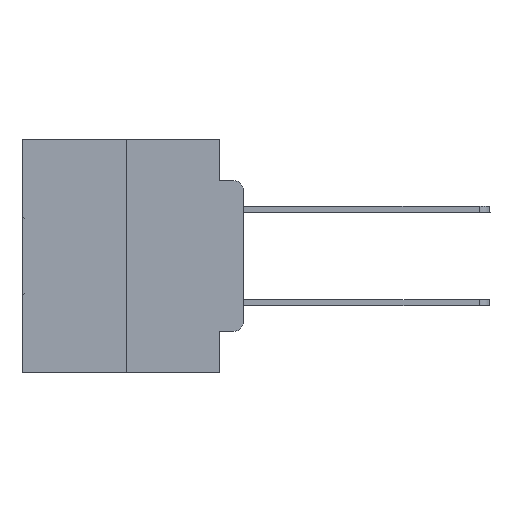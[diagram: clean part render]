
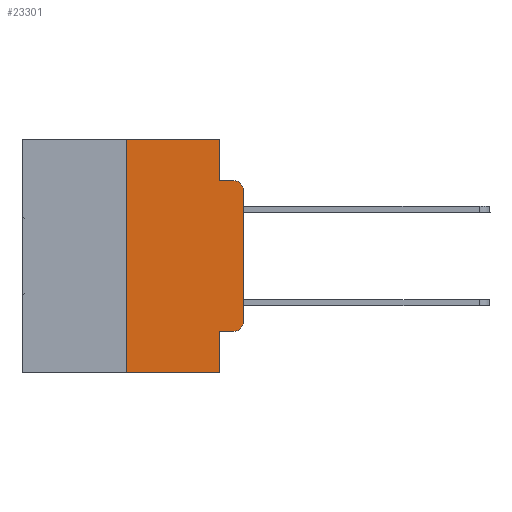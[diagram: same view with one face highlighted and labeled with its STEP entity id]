
A CAD part, left-side view. The second image highlights one B-rep face of the part: STEP entity #23301.
In plain terms, the highlighted planar face has unit normal (-1, 0, 0).
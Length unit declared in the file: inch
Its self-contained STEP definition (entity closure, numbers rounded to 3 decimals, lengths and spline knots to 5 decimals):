
#1292 = DIRECTION ( 'NONE',  ( 0., -1., 0. ) ) ;
#1364 = VECTOR ( 'NONE', #5255, 39.37008 ) ;
#1544 = AXIS2_PLACEMENT_3D ( 'NONE', #30973, #25988, #23099 ) ;
#1579 = VERTEX_POINT ( 'NONE', #13675 ) ;
#2563 = AXIS2_PLACEMENT_3D ( 'NONE', #10054, #17796, #10563 ) ;
#2618 = AXIS2_PLACEMENT_3D ( 'NONE', #30300, #25302, #14873 ) ;
#2721 = CARTESIAN_POINT ( 'NONE',  ( 0., 0.051, -0.4115 ) ) ;
#3250 = ORIENTED_EDGE ( 'NONE', *, *, #9442, .T. ) ;
#3460 = LINE ( 'NONE', #6198, #9876 ) ;
#3686 = VECTOR ( 'NONE', #20062, 39.37008 ) ;
#4103 = CARTESIAN_POINT ( 'NONE',  ( 0., 0.25, 0. ) ) ;
#4398 = LINE ( 'NONE', #9399, #3686 ) ;
#4515 = VERTEX_POINT ( 'NONE', #13543 ) ;
#4553 = CARTESIAN_POINT ( 'NONE',  ( 0., 0.473, 0. ) ) ;
#4576 = CARTESIAN_POINT ( 'NONE',  ( 0., 0.051, 0. ) ) ;
#4718 = EDGE_CURVE ( 'NONE', #13504, #28247, #10781, .T. ) ;
#4953 = CARTESIAN_POINT ( 'NONE',  ( 0., 0.051, -0.0885 ) ) ;
#5255 = DIRECTION ( 'NONE',  ( 0., 0., -1. ) ) ;
#5365 = CIRCLE ( 'NONE', #2618, 0.02 ) ;
#6198 = CARTESIAN_POINT ( 'NONE',  ( 0., 0.051, -0.0885 ) ) ;
#6205 = VECTOR ( 'NONE', #6881, 39.37008 ) ;
#6881 = DIRECTION ( 'NONE',  ( 0., 0., 1. ) ) ;
#7308 = DIRECTION ( 'NONE',  ( 0., -1., 0. ) ) ;
#7390 = EDGE_CURVE ( 'NONE', #4515, #11070, #23462, .T. ) ;
#7546 = EDGE_CURVE ( 'NONE', #19605, #24317, #3460, .T. ) ;
#8857 = LINE ( 'NONE', #2721, #30768 ) ;
#8997 = ORIENTED_EDGE ( 'NONE', *, *, #23970, .F. ) ;
#9291 = CARTESIAN_POINT ( 'NONE',  ( 0., 0.02, -0.4115 ) ) ;
#9399 = CARTESIAN_POINT ( 'NONE',  ( 0., 0.051, 0. ) ) ;
#9401 = ORIENTED_EDGE ( 'NONE', *, *, #23253, .T. ) ;
#9442 = EDGE_CURVE ( 'NONE', #4515, #11794, #11894, .T. ) ;
#9876 = VECTOR ( 'NONE', #13974, 39.37008 ) ;
#10054 = CARTESIAN_POINT ( 'NONE',  ( 0., 0.02, -0.3915 ) ) ;
#10563 = DIRECTION ( 'NONE',  ( 0., 0., -1. ) ) ;
#10646 = EDGE_CURVE ( 'NONE', #28247, #1579, #32330, .T. ) ;
#10781 = CIRCLE ( 'NONE', #2563, 0.02 ) ;
#11038 = DIRECTION ( 'NONE',  ( 0., 0., 1. ) ) ;
#11070 = VERTEX_POINT ( 'NONE', #4103 ) ;
#11562 = CARTESIAN_POINT ( 'NONE',  ( 0., 0., 0. ) ) ;
#11794 = VERTEX_POINT ( 'NONE', #12230 ) ;
#11894 = LINE ( 'NONE', #27161, #32446 ) ;
#12230 = CARTESIAN_POINT ( 'NONE',  ( 0., 0.051, -0.5 ) ) ;
#13504 = VERTEX_POINT ( 'NONE', #9291 ) ;
#13543 = CARTESIAN_POINT ( 'NONE',  ( 0., 0.25, -0.5 ) ) ;
#13675 = CARTESIAN_POINT ( 'NONE',  ( 0., 0., -0.1085 ) ) ;
#13974 = DIRECTION ( 'NONE',  ( 0., -1., 0. ) ) ;
#14487 = DIRECTION ( 'NONE',  ( 0., -1., 0. ) ) ;
#14700 = CARTESIAN_POINT ( 'NONE',  ( 0., 0.02, -0.0885 ) ) ;
#14769 = VECTOR ( 'NONE', #7308, 39.37008 ) ;
#14873 = DIRECTION ( 'NONE',  ( 0., 0., -1. ) ) ;
#15521 = VERTEX_POINT ( 'NONE', #4576 ) ;
#16601 = ORIENTED_EDGE ( 'NONE', *, *, #7390, .F. ) ;
#16636 = ORIENTED_EDGE ( 'NONE', *, *, #4718, .T. ) ;
#16859 = ORIENTED_EDGE ( 'NONE', *, *, #22783, .F. ) ;
#17007 = VECTOR ( 'NONE', #11038, 39.37008 ) ;
#17796 = DIRECTION ( 'NONE',  ( -1., 0., 0. ) ) ;
#17923 = EDGE_LOOP ( 'NONE', ( #21648, #9401, #26186, #16859, #8997, #16601, #3250, #23270, #21802, #16636 ) ) ;
#19605 = VERTEX_POINT ( 'NONE', #4953 ) ;
#20062 = DIRECTION ( 'NONE',  ( 0., 0., -1. ) ) ;
#20373 = LINE ( 'NONE', #4553, #14769 ) ;
#20856 = FACE_OUTER_BOUND ( 'NONE', #17923, .T. ) ;
#21648 = ORIENTED_EDGE ( 'NONE', *, *, #10646, .T. ) ;
#21802 = ORIENTED_EDGE ( 'NONE', *, *, #26856, .T. ) ;
#22783 = EDGE_CURVE ( 'NONE', #15521, #19605, #4398, .T. ) ;
#23099 = DIRECTION ( 'NONE',  ( 0., 0., -1. ) ) ;
#23253 = EDGE_CURVE ( 'NONE', #1579, #24317, #5365, .T. ) ;
#23270 = ORIENTED_EDGE ( 'NONE', *, *, #33643, .F. ) ;
#23301 = ADVANCED_FACE ( 'NONE', ( #20856 ), #33396, .F. ) ;
#23462 = LINE ( 'NONE', #33746, #17007 ) ;
#23970 = EDGE_CURVE ( 'NONE', #11070, #15521, #20373, .T. ) ;
#24164 = CARTESIAN_POINT ( 'NONE',  ( 0., 0.051, 0. ) ) ;
#24317 = VERTEX_POINT ( 'NONE', #14700 ) ;
#25302 = DIRECTION ( 'NONE',  ( -1., 0., 0. ) ) ;
#25988 = DIRECTION ( 'NONE',  ( 1., 0., 0. ) ) ;
#26186 = ORIENTED_EDGE ( 'NONE', *, *, #7546, .F. ) ;
#26353 = CARTESIAN_POINT ( 'NONE',  ( 0., 0., -0.3915 ) ) ;
#26856 = EDGE_CURVE ( 'NONE', #33352, #13504, #8857, .T. ) ;
#27161 = CARTESIAN_POINT ( 'NONE',  ( 0., 0.473, -0.5 ) ) ;
#28247 = VERTEX_POINT ( 'NONE', #26353 ) ;
#28612 = LINE ( 'NONE', #24164, #1364 ) ;
#29334 = CARTESIAN_POINT ( 'NONE',  ( 0., 0.051, -0.4115 ) ) ;
#30300 = CARTESIAN_POINT ( 'NONE',  ( 0., 0.02, -0.1085 ) ) ;
#30768 = VECTOR ( 'NONE', #1292, 39.37008 ) ;
#30973 = CARTESIAN_POINT ( 'NONE',  ( 0., 0.473, 0. ) ) ;
#32330 = LINE ( 'NONE', #11562, #6205 ) ;
#32446 = VECTOR ( 'NONE', #14487, 39.37008 ) ;
#33352 = VERTEX_POINT ( 'NONE', #29334 ) ;
#33396 = PLANE ( 'NONE',  #1544 ) ;
#33643 = EDGE_CURVE ( 'NONE', #33352, #11794, #28612, .T. ) ;
#33746 = CARTESIAN_POINT ( 'NONE',  ( 0., 0.25, 0. ) ) ;
